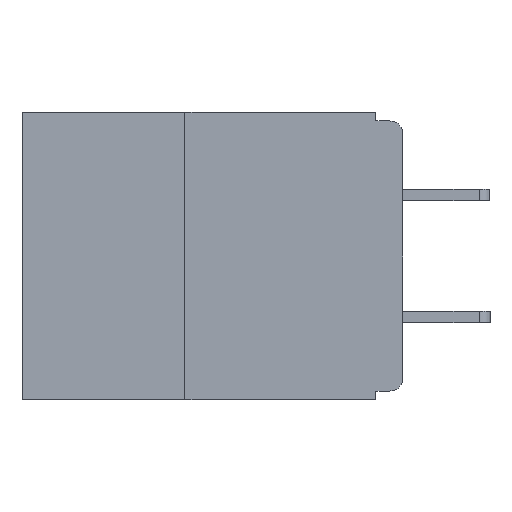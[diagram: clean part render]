
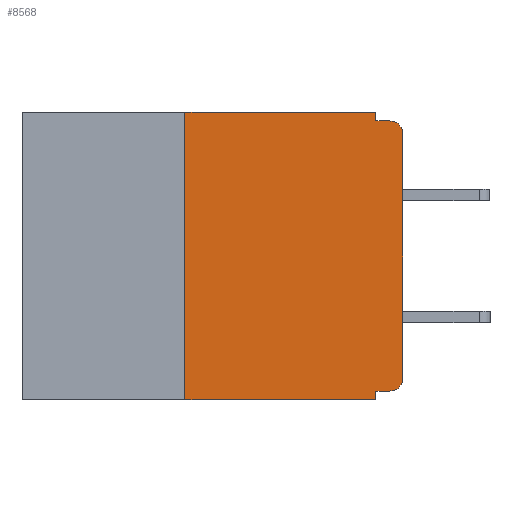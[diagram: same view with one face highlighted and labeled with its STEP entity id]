
A CAD part, left-side view. The second image highlights one B-rep face of the part: STEP entity #8568.
In plain terms, the highlighted planar face has unit normal (-1, 0, 0).
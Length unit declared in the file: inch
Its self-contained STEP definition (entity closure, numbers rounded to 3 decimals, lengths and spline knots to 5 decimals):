
#36 = DIRECTION ( 'NONE',  ( 0., 0., -1. ) ) ;
#667 = EDGE_CURVE ( 'NONE', #19035, #4433, #9437, .T. ) ;
#1124 = DIRECTION ( 'NONE',  ( 0., 1., 0. ) ) ;
#1497 = EDGE_CURVE ( 'NONE', #15682, #13385, #19159, .T. ) ;
#1759 = VECTOR ( 'NONE', #18844, 39.37008 ) ;
#1800 = VECTOR ( 'NONE', #7792, 39.37008 ) ;
#2964 = CARTESIAN_POINT ( 'NONE',  ( 0., 0.015, -0.32 ) ) ;
#3103 = CARTESIAN_POINT ( 'NONE',  ( 0., 0.015, -0.025 ) ) ;
#3127 = CARTESIAN_POINT ( 'NONE',  ( 0., 0.031, -0.32 ) ) ;
#3827 = ORIENTED_EDGE ( 'NONE', *, *, #25799, .F. ) ;
#4402 = DIRECTION ( 'NONE',  ( -1., 0., 0. ) ) ;
#4433 = VERTEX_POINT ( 'NONE', #22365 ) ;
#4575 = AXIS2_PLACEMENT_3D ( 'NONE', #32223, #19947, #4825 ) ;
#4597 = CARTESIAN_POINT ( 'NONE',  ( 0., 0.25, -0.33 ) ) ;
#4679 = CARTESIAN_POINT ( 'NONE',  ( 0., 0., -0.305 ) ) ;
#4825 = DIRECTION ( 'NONE',  ( 0., 0., -1. ) ) ;
#5180 = CARTESIAN_POINT ( 'NONE',  ( 0., 0., -0.01 ) ) ;
#5556 = DIRECTION ( 'NONE',  ( 0., -1., 0. ) ) ;
#5686 = DIRECTION ( 'NONE',  ( 0., 0., -1. ) ) ;
#6119 = EDGE_CURVE ( 'NONE', #15864, #15682, #13826, .T. ) ;
#7079 = ORIENTED_EDGE ( 'NONE', *, *, #14251, .F. ) ;
#7706 = VECTOR ( 'NONE', #31545, 39.37008 ) ;
#7792 = DIRECTION ( 'NONE',  ( 0., -1., 0. ) ) ;
#7970 = CARTESIAN_POINT ( 'NONE',  ( 0., 0., -0.025 ) ) ;
#8259 = ORIENTED_EDGE ( 'NONE', *, *, #28981, .F. ) ;
#8300 = ORIENTED_EDGE ( 'NONE', *, *, #30526, .T. ) ;
#8496 = VERTEX_POINT ( 'NONE', #4597 ) ;
#8506 = LINE ( 'NONE', #11541, #7706 ) ;
#8568 = ADVANCED_FACE ( 'NONE', ( #28212 ), #9864, .F. ) ;
#8819 = VERTEX_POINT ( 'NONE', #3127 ) ;
#9437 = LINE ( 'NONE', #24597, #1759 ) ;
#9472 = LINE ( 'NONE', #5180, #1800 ) ;
#9864 = PLANE ( 'NONE',  #4575 ) ;
#10646 = VERTEX_POINT ( 'NONE', #18324 ) ;
#10672 = CARTESIAN_POINT ( 'NONE',  ( 0., 0.437, 0. ) ) ;
#11541 = CARTESIAN_POINT ( 'NONE',  ( 0., 0.25, -0.33 ) ) ;
#11663 = VECTOR ( 'NONE', #14601, 39.37008 ) ;
#12804 = CARTESIAN_POINT ( 'NONE',  ( 0., 0.031, -0.33 ) ) ;
#13014 = LINE ( 'NONE', #12804, #13811 ) ;
#13120 = EDGE_CURVE ( 'NONE', #22025, #19035, #17763, .T. ) ;
#13385 = VERTEX_POINT ( 'NONE', #7970 ) ;
#13811 = VECTOR ( 'NONE', #36, 39.37008 ) ;
#13826 = CIRCLE ( 'NONE', #23272, 0.015 ) ;
#13918 = CIRCLE ( 'NONE', #14660, 0.015 ) ;
#13956 = CARTESIAN_POINT ( 'NONE',  ( 0., 0., 0. ) ) ;
#14251 = EDGE_CURVE ( 'NONE', #15864, #8819, #28112, .T. ) ;
#14601 = DIRECTION ( 'NONE',  ( 0., -1., 0. ) ) ;
#14660 = AXIS2_PLACEMENT_3D ( 'NONE', #3103, #20766, #5686 ) ;
#15031 = ORIENTED_EDGE ( 'NONE', *, *, #18317, .F. ) ;
#15055 = CARTESIAN_POINT ( 'NONE',  ( 0., 0.015, -0.305 ) ) ;
#15411 = ORIENTED_EDGE ( 'NONE', *, *, #6119, .T. ) ;
#15502 = DIRECTION ( 'NONE',  ( 0., 0., -1. ) ) ;
#15682 = VERTEX_POINT ( 'NONE', #4679 ) ;
#15864 = VERTEX_POINT ( 'NONE', #2964 ) ;
#16161 = ORIENTED_EDGE ( 'NONE', *, *, #667, .F. ) ;
#16501 = EDGE_LOOP ( 'NONE', ( #25924, #8300, #15031, #16161, #19240, #8259, #29727, #3827, #7079, #15411 ) ) ;
#16995 = CARTESIAN_POINT ( 'NONE',  ( 0., 0.031, -0.33 ) ) ;
#17763 = LINE ( 'NONE', #10672, #29327 ) ;
#18317 = EDGE_CURVE ( 'NONE', #4433, #10646, #9472, .T. ) ;
#18324 = CARTESIAN_POINT ( 'NONE',  ( 0., 0.015, -0.01 ) ) ;
#18844 = DIRECTION ( 'NONE',  ( 0., 0., -1. ) ) ;
#18893 = CARTESIAN_POINT ( 'NONE',  ( 0., 0., -0.32 ) ) ;
#19035 = VERTEX_POINT ( 'NONE', #25713 ) ;
#19133 = LINE ( 'NONE', #27000, #11663 ) ;
#19159 = LINE ( 'NONE', #13956, #30013 ) ;
#19240 = ORIENTED_EDGE ( 'NONE', *, *, #13120, .F. ) ;
#19947 = DIRECTION ( 'NONE',  ( 1., 0., 0. ) ) ;
#20766 = DIRECTION ( 'NONE',  ( -1., 0., 0. ) ) ;
#21499 = VECTOR ( 'NONE', #1124, 39.37008 ) ;
#22025 = VERTEX_POINT ( 'NONE', #28360 ) ;
#22365 = CARTESIAN_POINT ( 'NONE',  ( 0., 0.031, -0.01 ) ) ;
#23272 = AXIS2_PLACEMENT_3D ( 'NONE', #15055, #4402, #15502 ) ;
#24597 = CARTESIAN_POINT ( 'NONE',  ( 0., 0.031, 0. ) ) ;
#25713 = CARTESIAN_POINT ( 'NONE',  ( 0., 0.031, 0. ) ) ;
#25799 = EDGE_CURVE ( 'NONE', #8819, #30695, #13014, .T. ) ;
#25924 = ORIENTED_EDGE ( 'NONE', *, *, #1497, .T. ) ;
#27000 = CARTESIAN_POINT ( 'NONE',  ( 0., 0.437, -0.33 ) ) ;
#28112 = LINE ( 'NONE', #18893, #21499 ) ;
#28212 = FACE_OUTER_BOUND ( 'NONE', #16501, .T. ) ;
#28360 = CARTESIAN_POINT ( 'NONE',  ( 0., 0.25, 0. ) ) ;
#28435 = EDGE_CURVE ( 'NONE', #8496, #30695, #19133, .T. ) ;
#28981 = EDGE_CURVE ( 'NONE', #8496, #22025, #8506, .T. ) ;
#29327 = VECTOR ( 'NONE', #5556, 39.37008 ) ;
#29418 = DIRECTION ( 'NONE',  ( 0., 0., 1. ) ) ;
#29727 = ORIENTED_EDGE ( 'NONE', *, *, #28435, .T. ) ;
#30013 = VECTOR ( 'NONE', #29418, 39.37008 ) ;
#30526 = EDGE_CURVE ( 'NONE', #13385, #10646, #13918, .T. ) ;
#30695 = VERTEX_POINT ( 'NONE', #16995 ) ;
#31545 = DIRECTION ( 'NONE',  ( 0., 0., 1. ) ) ;
#32223 = CARTESIAN_POINT ( 'NONE',  ( 0., 0.437, 0. ) ) ;
